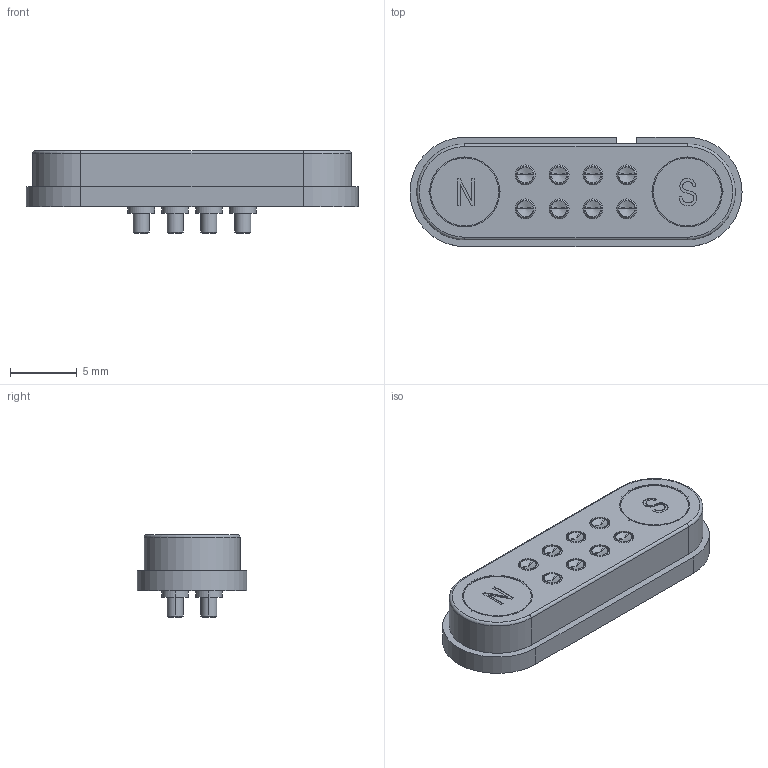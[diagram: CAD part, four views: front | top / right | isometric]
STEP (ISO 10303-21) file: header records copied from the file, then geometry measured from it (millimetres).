
FILE_DESCRIPTION (( 'STEP AP214' ), '1' );
FILE_NAME ('686B0822250210E.STEP', '2023-04-27T17:17:30', ( '' ), ( '' ), 'SwSTEP 2.0', 'SolidWorks 2020', '' );
FILE_SCHEMA (( 'AUTOMOTIVE_DESIGN' ));
Length unit declared in the file: millimetre
Products named in the file (1): 686B0822250210E
Bounding box: 24.9 x 8.2 x 6.2 mm (x, y, z)
Volume: 702.9 mm3; surface area: 962.8 mm2
Topology: 3 solids, 3 shells, 208 faces, 480 edges, 296 vertices
Faces by surface type: cone 64, cylinder 64, plane 52, torus 14, bspline 14
Entity records: 8880 total; most frequent: CARTESIAN_POINT 1799, DIRECTION 1060, ORIENTED_EDGE 928, EDGE_CURVE 464, AXIS2_PLACEMENT_3D 429, VERTEX_POINT 296, EDGE_LOOP 246, CIRCLE 234
